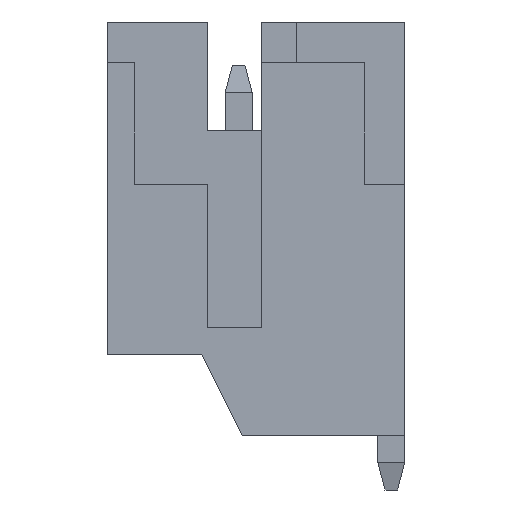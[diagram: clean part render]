
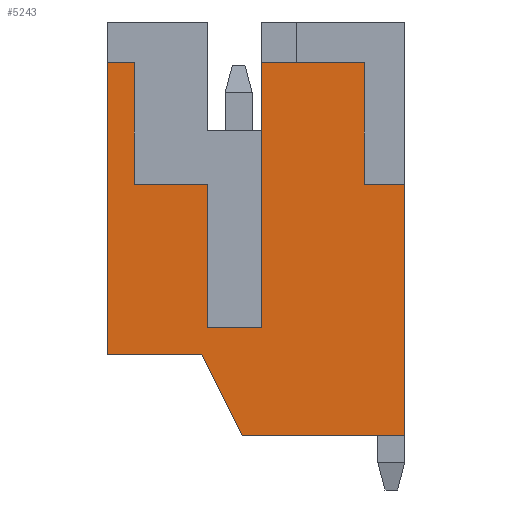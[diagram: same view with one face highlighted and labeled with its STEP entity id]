
A CAD part, left-side view. The second image highlights one B-rep face of the part: STEP entity #5243.
In plain terms, the highlighted planar face has unit normal (-1, 0, 0).
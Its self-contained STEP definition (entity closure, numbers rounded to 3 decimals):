
#51 = LINE ( 'NONE', #3632, #6122 ) ;
#113 = VERTEX_POINT ( 'NONE', #3148 ) ;
#130 = VECTOR ( 'NONE', #298, 1000. ) ;
#144 = DIRECTION ( 'NONE',  ( 0., 0., -1. ) ) ;
#216 = CARTESIAN_POINT ( 'NONE',  ( -3., -2.32, 3.15 ) ) ;
#230 = LINE ( 'NONE', #6714, #3701 ) ;
#298 = DIRECTION ( 'NONE',  ( 0., 0., -1. ) ) ;
#486 = CARTESIAN_POINT ( 'NONE',  ( -3., 0.58, 3.15 ) ) ;
#501 = VECTOR ( 'NONE', #6588, 1000. ) ;
#503 = CARTESIAN_POINT ( 'NONE',  ( -3., 2.43, 5.4 ) ) ;
#543 = CARTESIAN_POINT ( 'NONE',  ( -3., -0.42, 5.4 ) ) ;
#664 = LINE ( 'NONE', #5175, #1683 ) ;
#665 = CARTESIAN_POINT ( 'NONE',  ( -3., -2.32, 5.4 ) ) ;
#715 = VECTOR ( 'NONE', #144, 1000. ) ;
#780 = CARTESIAN_POINT ( 'NONE',  ( -3., -0.07, -1.5 ) ) ;
#802 = VERTEX_POINT ( 'NONE', #6678 ) ;
#808 = FACE_OUTER_BOUND ( 'NONE', #6195, .T. ) ;
#831 = DIRECTION ( 'NONE',  ( 0., 1., 0. ) ) ;
#950 = DIRECTION ( 'NONE',  ( 0., 0., 1. ) ) ;
#999 = CARTESIAN_POINT ( 'NONE',  ( -3., 2.43, 0. ) ) ;
#1106 = LINE ( 'NONE', #6962, #2710 ) ;
#1136 = DIRECTION ( 'NONE',  ( 0., -1., 0. ) ) ;
#1227 = LINE ( 'NONE', #3513, #6781 ) ;
#1315 = VERTEX_POINT ( 'NONE', #2652 ) ;
#1521 = ORIENTED_EDGE ( 'NONE', *, *, #3138, .F. ) ;
#1589 = ORIENTED_EDGE ( 'NONE', *, *, #3753, .T. ) ;
#1591 = VERTEX_POINT ( 'NONE', #216 ) ;
#1592 = AXIS2_PLACEMENT_3D ( 'NONE', #3864, #2226, #1136 ) ;
#1683 = VECTOR ( 'NONE', #5231, 1000. ) ;
#1694 = EDGE_CURVE ( 'NONE', #4297, #3683, #230, .T. ) ;
#1848 = DIRECTION ( 'NONE',  ( 0., 0., -1. ) ) ;
#2110 = LINE ( 'NONE', #3449, #3708 ) ;
#2115 = VERTEX_POINT ( 'NONE', #665 ) ;
#2159 = EDGE_CURVE ( 'NONE', #4312, #1315, #5116, .T. ) ;
#2173 = VECTOR ( 'NONE', #950, 1000. ) ;
#2195 = ORIENTED_EDGE ( 'NONE', *, *, #4444, .T. ) ;
#2226 = DIRECTION ( 'NONE',  ( -1., 0., 0. ) ) ;
#2240 = PLANE ( 'NONE',  #1592 ) ;
#2254 = LINE ( 'NONE', #3402, #715 ) ;
#2255 = EDGE_CURVE ( 'NONE', #802, #2392, #2846, .T. ) ;
#2392 = VERTEX_POINT ( 'NONE', #6921 ) ;
#2435 = VECTOR ( 'NONE', #5171, 1000. ) ;
#2537 = CARTESIAN_POINT ( 'NONE',  ( -3., 1.93, 3.15 ) ) ;
#2579 = CARTESIAN_POINT ( 'NONE',  ( -3., -3.07, 3.15 ) ) ;
#2610 = VECTOR ( 'NONE', #4628, 1000. ) ;
#2652 = CARTESIAN_POINT ( 'NONE',  ( -3., 0.58, 0.5 ) ) ;
#2710 = VECTOR ( 'NONE', #5348, 1000. ) ;
#2835 = ORIENTED_EDGE ( 'NONE', *, *, #2159, .F. ) ;
#2846 = LINE ( 'NONE', #2537, #2173 ) ;
#2892 = CARTESIAN_POINT ( 'NONE',  ( -3., -0.42, 0.5 ) ) ;
#2919 = EDGE_CURVE ( 'NONE', #802, #4312, #5999, .T. ) ;
#3138 = EDGE_CURVE ( 'NONE', #1591, #3683, #664, .T. ) ;
#3148 = CARTESIAN_POINT ( 'NONE',  ( -3., 0.68, 0. ) ) ;
#3390 = EDGE_CURVE ( 'NONE', #6280, #5437, #2110, .T. ) ;
#3392 = ORIENTED_EDGE ( 'NONE', *, *, #5186, .T. ) ;
#3402 = CARTESIAN_POINT ( 'NONE',  ( -3., -0.42, 6.15 ) ) ;
#3438 = LINE ( 'NONE', #780, #2435 ) ;
#3449 = CARTESIAN_POINT ( 'NONE',  ( -3., 2.43, 6.15 ) ) ;
#3450 = DIRECTION ( 'NONE',  ( 0., -1., 0. ) ) ;
#3511 = ORIENTED_EDGE ( 'NONE', *, *, #6245, .T. ) ;
#3513 = CARTESIAN_POINT ( 'NONE',  ( -3., -3.07, 5.4 ) ) ;
#3632 = CARTESIAN_POINT ( 'NONE',  ( -3., -2.32, 3.15 ) ) ;
#3683 = VERTEX_POINT ( 'NONE', #2579 ) ;
#3701 = VECTOR ( 'NONE', #5154, 1000. ) ;
#3708 = VECTOR ( 'NONE', #1848, 1000. ) ;
#3729 = CARTESIAN_POINT ( 'NONE',  ( -3., -3.07, -1.5 ) ) ;
#3753 = EDGE_CURVE ( 'NONE', #5437, #113, #1106, .T. ) ;
#3792 = VERTEX_POINT ( 'NONE', #543 ) ;
#3857 = ORIENTED_EDGE ( 'NONE', *, *, #4163, .T. ) ;
#3864 = CARTESIAN_POINT ( 'NONE',  ( -3., 0., 0. ) ) ;
#4103 = VECTOR ( 'NONE', #5347, 1000. ) ;
#4163 = EDGE_CURVE ( 'NONE', #5981, #4297, #6380, .T. ) ;
#4297 = VERTEX_POINT ( 'NONE', #3729 ) ;
#4312 = VERTEX_POINT ( 'NONE', #486 ) ;
#4406 = ORIENTED_EDGE ( 'NONE', *, *, #4803, .T. ) ;
#4444 = EDGE_CURVE ( 'NONE', #2392, #6280, #6887, .T. ) ;
#4603 = LINE ( 'NONE', #6934, #4103 ) ;
#4628 = DIRECTION ( 'NONE',  ( 0., 1., 0. ) ) ;
#4674 = EDGE_CURVE ( 'NONE', #113, #5981, #3438, .T. ) ;
#4727 = ORIENTED_EDGE ( 'NONE', *, *, #4674, .T. ) ;
#4803 = EDGE_CURVE ( 'NONE', #1591, #2115, #51, .T. ) ;
#5074 = CARTESIAN_POINT ( 'NONE',  ( -3., -0.42, 3.15 ) ) ;
#5116 = LINE ( 'NONE', #6728, #130 ) ;
#5154 = DIRECTION ( 'NONE',  ( 0., 0., 1. ) ) ;
#5171 = DIRECTION ( 'NONE',  ( 0., -0.447, -0.894 ) ) ;
#5175 = CARTESIAN_POINT ( 'NONE',  ( -3., -2.32, 3.15 ) ) ;
#5186 = EDGE_CURVE ( 'NONE', #3792, #6075, #2254, .T. ) ;
#5215 = ORIENTED_EDGE ( 'NONE', *, *, #2255, .T. ) ;
#5224 = ORIENTED_EDGE ( 'NONE', *, *, #2919, .F. ) ;
#5231 = DIRECTION ( 'NONE',  ( 0., -1., 0. ) ) ;
#5243 = ADVANCED_FACE ( 'NONE', ( #808 ), #2240, .T. ) ;
#5347 = DIRECTION ( 'NONE',  ( 0., -1., 0. ) ) ;
#5348 = DIRECTION ( 'NONE',  ( 0., -1., 0. ) ) ;
#5420 = EDGE_CURVE ( 'NONE', #1315, #6075, #4603, .T. ) ;
#5437 = VERTEX_POINT ( 'NONE', #999 ) ;
#5502 = CARTESIAN_POINT ( 'NONE',  ( -3., -0.07, -1.5 ) ) ;
#5600 = ORIENTED_EDGE ( 'NONE', *, *, #5420, .F. ) ;
#5697 = ORIENTED_EDGE ( 'NONE', *, *, #1694, .T. ) ;
#5981 = VERTEX_POINT ( 'NONE', #5502 ) ;
#5999 = LINE ( 'NONE', #5074, #6076 ) ;
#6075 = VERTEX_POINT ( 'NONE', #2892 ) ;
#6076 = VECTOR ( 'NONE', #3450, 1000. ) ;
#6122 = VECTOR ( 'NONE', #6332, 1000. ) ;
#6195 = EDGE_LOOP ( 'NONE', ( #2195, #6234, #1589, #4727, #3857, #5697, #1521, #4406, #3511, #3392, #5600, #2835, #5224, #5215 ) ) ;
#6234 = ORIENTED_EDGE ( 'NONE', *, *, #3390, .T. ) ;
#6245 = EDGE_CURVE ( 'NONE', #2115, #3792, #1227, .T. ) ;
#6280 = VERTEX_POINT ( 'NONE', #503 ) ;
#6332 = DIRECTION ( 'NONE',  ( 0., 0., 1. ) ) ;
#6380 = LINE ( 'NONE', #6725, #501 ) ;
#6588 = DIRECTION ( 'NONE',  ( 0., -1., 0. ) ) ;
#6678 = CARTESIAN_POINT ( 'NONE',  ( -3., 1.93, 3.15 ) ) ;
#6714 = CARTESIAN_POINT ( 'NONE',  ( -3., -3.07, 6.15 ) ) ;
#6725 = CARTESIAN_POINT ( 'NONE',  ( -3., -3.07, -1.5 ) ) ;
#6728 = CARTESIAN_POINT ( 'NONE',  ( -3., 0.58, 3.15 ) ) ;
#6736 = CARTESIAN_POINT ( 'NONE',  ( -3., -3.07, 5.4 ) ) ;
#6781 = VECTOR ( 'NONE', #831, 1000. ) ;
#6887 = LINE ( 'NONE', #6736, #2610 ) ;
#6921 = CARTESIAN_POINT ( 'NONE',  ( -3., 1.93, 5.4 ) ) ;
#6934 = CARTESIAN_POINT ( 'NONE',  ( -3., -0.42, 0.5 ) ) ;
#6962 = CARTESIAN_POINT ( 'NONE',  ( -3., 2.43, 0. ) ) ;
